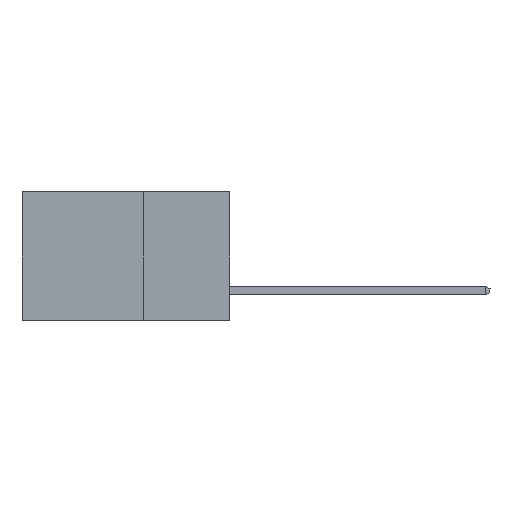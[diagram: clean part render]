
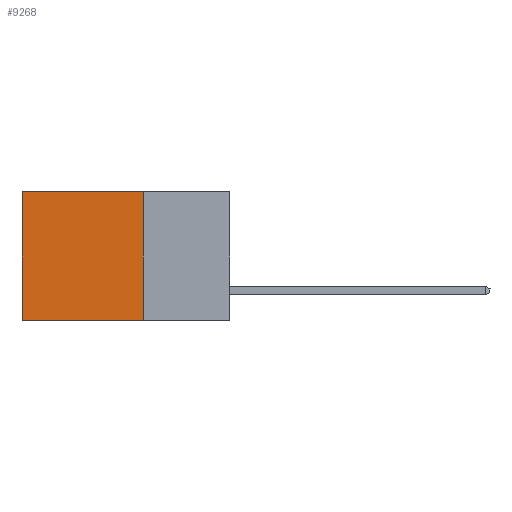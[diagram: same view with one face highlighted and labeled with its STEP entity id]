
A CAD part, left-side view. The second image highlights one B-rep face of the part: STEP entity #9268.
In plain terms, the highlighted planar face has unit normal (-1, 0, 0).
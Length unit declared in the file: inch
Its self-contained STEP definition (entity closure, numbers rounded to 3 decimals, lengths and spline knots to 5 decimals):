
#776 = VERTEX_POINT ( 'NONE', #13293 ) ;
#905 = CARTESIAN_POINT ( 'NONE',  ( 0.2615, 0.25, 0. ) ) ;
#1411 = CARTESIAN_POINT ( 'NONE',  ( 0.2615, 0.25, -0.37 ) ) ;
#1544 = CARTESIAN_POINT ( 'NONE',  ( 0.2615, 0.6, -0.37 ) ) ;
#2066 = EDGE_CURVE ( 'NONE', #14846, #7909, #19290, .T. ) ;
#2805 = DIRECTION ( 'NONE',  ( 1., 0., 0. ) ) ;
#2933 = VERTEX_POINT ( 'NONE', #905 ) ;
#5644 = EDGE_CURVE ( 'NONE', #776, #7909, #17648, .T. ) ;
#6395 = EDGE_CURVE ( 'NONE', #2933, #14846, #15862, .T. ) ;
#6808 = VECTOR ( 'NONE', #20882, 39.37008 ) ;
#7548 = ORIENTED_EDGE ( 'NONE', *, *, #2066, .T. ) ;
#7909 = VERTEX_POINT ( 'NONE', #9003 ) ;
#9003 = CARTESIAN_POINT ( 'NONE',  ( 0.2615, 0.6, -0.37 ) ) ;
#9268 = ADVANCED_FACE ( 'NONE', ( #10890 ), #10789, .F. ) ;
#9637 = DIRECTION ( 'NONE',  ( 0., 1., 0. ) ) ;
#10484 = ORIENTED_EDGE ( 'NONE', *, *, #10829, .F. ) ;
#10789 = PLANE ( 'NONE',  #10812 ) ;
#10812 = AXIS2_PLACEMENT_3D ( 'NONE', #17449, #2805, #17343 ) ;
#10829 = EDGE_CURVE ( 'NONE', #2933, #776, #17212, .T. ) ;
#10890 = FACE_OUTER_BOUND ( 'NONE', #17382, .T. ) ;
#10976 = DIRECTION ( 'NONE',  ( 0., 0., -1. ) ) ;
#11017 = CARTESIAN_POINT ( 'NONE',  ( 0.2615, 0.25, 0. ) ) ;
#12602 = DIRECTION ( 'NONE',  ( 0., 1., 0. ) ) ;
#12909 = ORIENTED_EDGE ( 'NONE', *, *, #5644, .F. ) ;
#13293 = CARTESIAN_POINT ( 'NONE',  ( 0.2615, 0.25, -0.37 ) ) ;
#13614 = VECTOR ( 'NONE', #10976, 39.37008 ) ;
#13780 = ORIENTED_EDGE ( 'NONE', *, *, #6395, .T. ) ;
#13843 = VECTOR ( 'NONE', #12602, 39.37008 ) ;
#14846 = VERTEX_POINT ( 'NONE', #20694 ) ;
#15862 = LINE ( 'NONE', #11017, #15888 ) ;
#15888 = VECTOR ( 'NONE', #9637, 39.37008 ) ;
#17212 = LINE ( 'NONE', #20435, #13614 ) ;
#17343 = DIRECTION ( 'NONE',  ( 0., 0., -1. ) ) ;
#17382 = EDGE_LOOP ( 'NONE', ( #7548, #12909, #10484, #13780 ) ) ;
#17449 = CARTESIAN_POINT ( 'NONE',  ( 0.2615, 0.25, -0.37 ) ) ;
#17648 = LINE ( 'NONE', #1411, #13843 ) ;
#19290 = LINE ( 'NONE', #1544, #6808 ) ;
#20435 = CARTESIAN_POINT ( 'NONE',  ( 0.2615, 0.25, -0.37 ) ) ;
#20694 = CARTESIAN_POINT ( 'NONE',  ( 0.2615, 0.6, 0. ) ) ;
#20882 = DIRECTION ( 'NONE',  ( 0., 0., -1. ) ) ;
